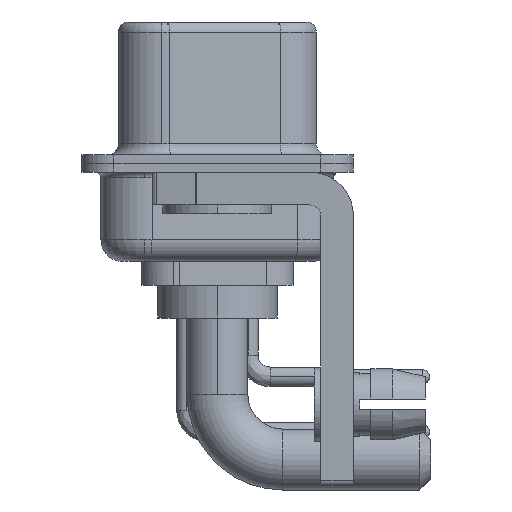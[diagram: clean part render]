
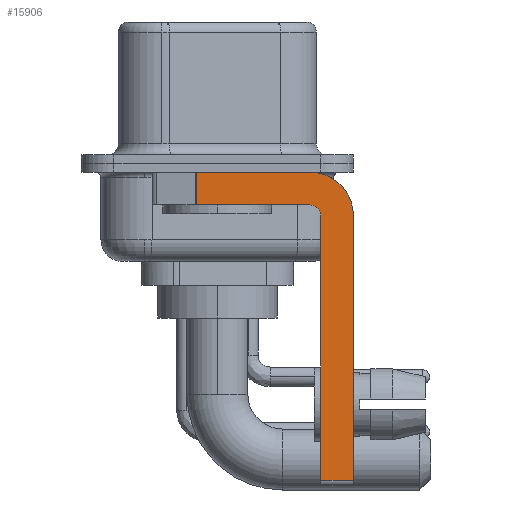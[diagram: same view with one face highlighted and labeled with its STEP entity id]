
A CAD part, left-side view. The second image highlights one B-rep face of the part: STEP entity #15906.
In plain terms, the highlighted planar face has unit normal (-1, 0, 0).
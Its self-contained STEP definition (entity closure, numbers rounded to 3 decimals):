
#701 = EDGE_LOOP ( 'NONE', ( #4985, #20769, #28949, #28691, #16316, #5547, #12252, #2747 ) ) ;
#795 = VECTOR ( 'NONE', #5501, 1000. ) ;
#1086 = CARTESIAN_POINT ( 'NONE',  ( -2.9, -4.75, -14.8 ) ) ;
#1424 = CARTESIAN_POINT ( 'NONE',  ( -2.9, -4.25, -2.4 ) ) ;
#1569 = PLANE ( 'NONE',  #15540 ) ;
#2014 = VECTOR ( 'NONE', #21476, 1000. ) ;
#2747 = ORIENTED_EDGE ( 'NONE', *, *, #14711, .F. ) ;
#3014 = LINE ( 'NONE', #14504, #19053 ) ;
#3061 = EDGE_CURVE ( 'NONE', #10002, #12525, #25659, .T. ) ;
#4487 = CARTESIAN_POINT ( 'NONE',  ( -2.9, 0.978, -1.9 ) ) ;
#4694 = CARTESIAN_POINT ( 'NONE',  ( -2.9, -4.25, -0.4 ) ) ;
#4985 = ORIENTED_EDGE ( 'NONE', *, *, #5647, .F. ) ;
#5195 = CARTESIAN_POINT ( 'NONE',  ( -2.9, 0.978, -1.9 ) ) ;
#5247 = VECTOR ( 'NONE', #21930, 1000. ) ;
#5258 = DIRECTION ( 'NONE',  ( 0., 0., 1. ) ) ;
#5415 = VECTOR ( 'NONE', #5258, 1000. ) ;
#5501 = DIRECTION ( 'NONE',  ( 0., 0., -1. ) ) ;
#5547 = ORIENTED_EDGE ( 'NONE', *, *, #25237, .T. ) ;
#5647 = EDGE_CURVE ( 'NONE', #20775, #16423, #28976, .T. ) ;
#6885 = EDGE_CURVE ( 'NONE', #15058, #10377, #21284, .T. ) ;
#7365 = VERTEX_POINT ( 'NONE', #4487 ) ;
#7684 = DIRECTION ( 'NONE',  ( 0., 0., -1. ) ) ;
#9081 = CARTESIAN_POINT ( 'NONE',  ( -2.9, 0.978, -0.4 ) ) ;
#9150 = CARTESIAN_POINT ( 'NONE',  ( -2.9, -6.25, -2.4 ) ) ;
#9933 = CARTESIAN_POINT ( 'NONE',  ( -2.9, -4.25, -2.4 ) ) ;
#9980 = CARTESIAN_POINT ( 'NONE',  ( -2.9, -4.75, -14.55 ) ) ;
#10002 = VERTEX_POINT ( 'NONE', #12425 ) ;
#10377 = VERTEX_POINT ( 'NONE', #18953 ) ;
#12229 = DIRECTION ( 'NONE',  ( 0., -1., 0. ) ) ;
#12252 = ORIENTED_EDGE ( 'NONE', *, *, #6885, .F. ) ;
#12279 = LINE ( 'NONE', #23780, #2014 ) ;
#12425 = CARTESIAN_POINT ( 'NONE',  ( -2.9, -4.75, -2.4 ) ) ;
#12525 = VERTEX_POINT ( 'NONE', #18960 ) ;
#14504 = CARTESIAN_POINT ( 'NONE',  ( -2.9, -4.25, -14.55 ) ) ;
#14711 = EDGE_CURVE ( 'NONE', #16423, #15058, #27722, .T. ) ;
#14766 = EDGE_CURVE ( 'NONE', #20775, #7365, #23903, .T. ) ;
#15058 = VERTEX_POINT ( 'NONE', #9150 ) ;
#15136 = DIRECTION ( 'NONE',  ( 0., 0., -1. ) ) ;
#15540 = AXIS2_PLACEMENT_3D ( 'NONE', #1424, #24429, #29474 ) ;
#15579 = DIRECTION ( 'NONE',  ( 0., 0., 1. ) ) ;
#15906 = ADVANCED_FACE ( 'NONE', ( #22434 ), #1569, .F. ) ;
#16316 = ORIENTED_EDGE ( 'NONE', *, *, #24863, .F. ) ;
#16423 = VERTEX_POINT ( 'NONE', #4694 ) ;
#16935 = AXIS2_PLACEMENT_3D ( 'NONE', #9933, #17268, #15136 ) ;
#17268 = DIRECTION ( 'NONE',  ( 1., 0., 0. ) ) ;
#17882 = CARTESIAN_POINT ( 'NONE',  ( -2.9, -4.25, -2.4 ) ) ;
#18953 = CARTESIAN_POINT ( 'NONE',  ( -2.9, -6.25, -14.55 ) ) ;
#18960 = CARTESIAN_POINT ( 'NONE',  ( -2.9, -4.25, -1.9 ) ) ;
#19007 = CARTESIAN_POINT ( 'NONE',  ( -2.9, -6.25, -2.4 ) ) ;
#19053 = VECTOR ( 'NONE', #12229, 1000. ) ;
#20769 = ORIENTED_EDGE ( 'NONE', *, *, #14766, .T. ) ;
#20775 = VERTEX_POINT ( 'NONE', #9081 ) ;
#20799 = VERTEX_POINT ( 'NONE', #9980 ) ;
#21284 = LINE ( 'NONE', #19007, #23436 ) ;
#21476 = DIRECTION ( 'NONE',  ( 0., 1., 0. ) ) ;
#21930 = DIRECTION ( 'NONE',  ( 0., -1., 0. ) ) ;
#22434 = FACE_OUTER_BOUND ( 'NONE', #701, .T. ) ;
#23101 = DIRECTION ( 'NONE',  ( -1., 0., 0. ) ) ;
#23436 = VECTOR ( 'NONE', #7684, 1000. ) ;
#23780 = CARTESIAN_POINT ( 'NONE',  ( -2.9, -4.25, -1.9 ) ) ;
#23903 = LINE ( 'NONE', #5195, #795 ) ;
#24429 = DIRECTION ( 'NONE',  ( 1., 0., 0. ) ) ;
#24863 = EDGE_CURVE ( 'NONE', #20799, #10002, #29152, .T. ) ;
#25237 = EDGE_CURVE ( 'NONE', #20799, #10377, #3014, .T. ) ;
#25659 = CIRCLE ( 'NONE', #27596, 0.5 ) ;
#27132 = CARTESIAN_POINT ( 'NONE',  ( -2.9, 3., -0.4 ) ) ;
#27571 = EDGE_CURVE ( 'NONE', #12525, #7365, #12279, .T. ) ;
#27596 = AXIS2_PLACEMENT_3D ( 'NONE', #17882, #23101, #15579 ) ;
#27722 = CIRCLE ( 'NONE', #16935, 2. ) ;
#28691 = ORIENTED_EDGE ( 'NONE', *, *, #3061, .F. ) ;
#28949 = ORIENTED_EDGE ( 'NONE', *, *, #27571, .F. ) ;
#28976 = LINE ( 'NONE', #27132, #5247 ) ;
#29152 = LINE ( 'NONE', #1086, #5415 ) ;
#29474 = DIRECTION ( 'NONE',  ( 0., 0., -1. ) ) ;
